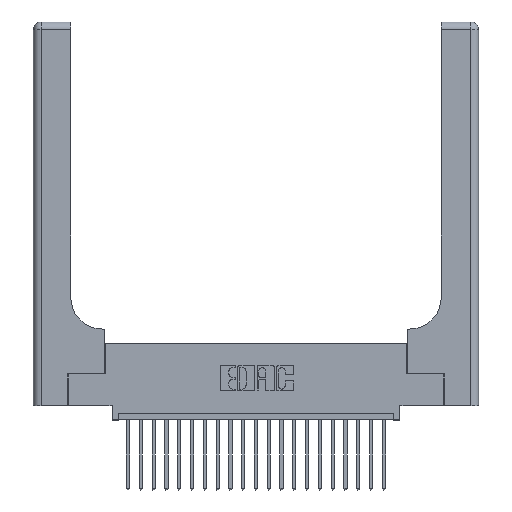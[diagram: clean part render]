
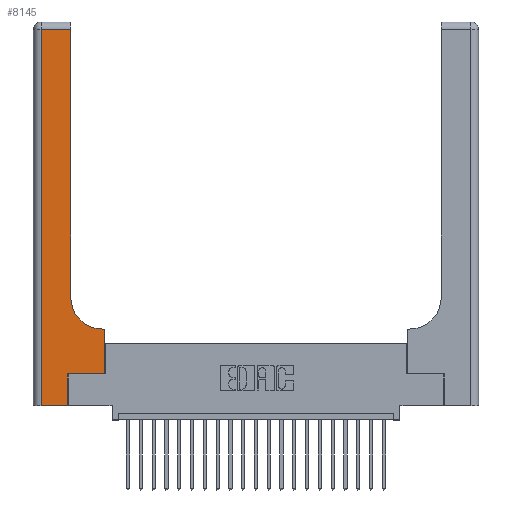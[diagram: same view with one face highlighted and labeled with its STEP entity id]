
A CAD part, top view. The second image highlights one B-rep face of the part: STEP entity #8145.
In plain terms, the highlighted planar face has unit normal (0, 0, 1).
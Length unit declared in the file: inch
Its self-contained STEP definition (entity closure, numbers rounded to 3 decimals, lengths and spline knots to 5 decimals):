
#532 = EDGE_CURVE ( 'NONE', #6200, #13840, #13976, .T. ) ;
#576 = VECTOR ( 'NONE', #5150, 39.37008 ) ;
#609 = CIRCLE ( 'NONE', #21544, 0.25 ) ;
#1213 = EDGE_CURVE ( 'NONE', #2058, #22626, #7510, .T. ) ;
#1431 = VECTOR ( 'NONE', #8332, 39.37008 ) ;
#1507 = DIRECTION ( 'NONE',  ( -1., 0., 0. ) ) ;
#1637 = CARTESIAN_POINT ( 'NONE',  ( 0.06, 0., 0.37 ) ) ;
#1995 = DIRECTION ( 'NONE',  ( 0., 1., 0. ) ) ;
#1996 = LINE ( 'NONE', #12170, #1431 ) ;
#2058 = VERTEX_POINT ( 'NONE', #10791 ) ;
#2705 = VECTOR ( 'NONE', #20865, 39.37008 ) ;
#3400 = DIRECTION ( 'NONE',  ( 0., -1., 0. ) ) ;
#3778 = EDGE_CURVE ( 'NONE', #13840, #16479, #17340, .T. ) ;
#4126 = FACE_OUTER_BOUND ( 'NONE', #4736, .T. ) ;
#4736 = EDGE_LOOP ( 'NONE', ( #5119, #21849, #23039, #14675, #19238, #20548, #11868, #14388, #14847 ) ) ;
#5119 = ORIENTED_EDGE ( 'NONE', *, *, #18127, .T. ) ;
#5150 = DIRECTION ( 'NONE',  ( 0., 1., 0. ) ) ;
#5796 = VECTOR ( 'NONE', #3400, 39.37008 ) ;
#5924 = CARTESIAN_POINT ( 'NONE',  ( 0.06, 2.94, 0.37 ) ) ;
#6200 = VERTEX_POINT ( 'NONE', #5924 ) ;
#6630 = DIRECTION ( 'NONE',  ( 1., 0., 0. ) ) ;
#7039 = CARTESIAN_POINT ( 'NONE',  ( 0.5585, 0.6, 0.37 ) ) ;
#7337 = VERTEX_POINT ( 'NONE', #23247 ) ;
#7508 = CARTESIAN_POINT ( 'NONE',  ( 0.06, 3., 0.37 ) ) ;
#7510 = LINE ( 'NONE', #7542, #11267 ) ;
#7542 = CARTESIAN_POINT ( 'NONE',  ( 0.5585, 0.25, 0.37 ) ) ;
#7878 = LINE ( 'NONE', #15792, #576 ) ;
#8145 = ADVANCED_FACE ( 'NONE', ( #4126 ), #12210, .F. ) ;
#8175 = VERTEX_POINT ( 'NONE', #12602 ) ;
#8332 = DIRECTION ( 'NONE',  ( -1., 0., 0. ) ) ;
#8670 = VECTOR ( 'NONE', #23509, 39.37008 ) ;
#9211 = VERTEX_POINT ( 'NONE', #11622 ) ;
#9389 = DIRECTION ( 'NONE',  ( 0., 1., 0. ) ) ;
#10196 = EDGE_CURVE ( 'NONE', #16479, #9211, #15954, .T. ) ;
#10234 = EDGE_CURVE ( 'NONE', #7337, #6200, #22549, .T. ) ;
#10723 = VECTOR ( 'NONE', #1507, 39.37008 ) ;
#10791 = CARTESIAN_POINT ( 'NONE',  ( 0.5585, 0.25, 0.37 ) ) ;
#10989 = VECTOR ( 'NONE', #1995, 39.37008 ) ;
#11267 = VECTOR ( 'NONE', #9389, 39.37008 ) ;
#11318 = CARTESIAN_POINT ( 'NONE',  ( 0.269, 0.25, 0.37 ) ) ;
#11323 = CARTESIAN_POINT ( 'NONE',  ( 0., 0., 0.37 ) ) ;
#11425 = CARTESIAN_POINT ( 'NONE',  ( 0.269, 0., 0.37 ) ) ;
#11622 = CARTESIAN_POINT ( 'NONE',  ( 0.269, 0.25, 0.37 ) ) ;
#11868 = ORIENTED_EDGE ( 'NONE', *, *, #1213, .T. ) ;
#11921 = AXIS2_PLACEMENT_3D ( 'NONE', #15779, #23682, #19747 ) ;
#12170 = CARTESIAN_POINT ( 'NONE',  ( 0.2915, 0.6, 0.37 ) ) ;
#12210 = PLANE ( 'NONE',  #11921 ) ;
#12602 = CARTESIAN_POINT ( 'NONE',  ( 0.2915, 0.85, 0.37 ) ) ;
#13005 = CARTESIAN_POINT ( 'NONE',  ( 0.269, 0., 0.37 ) ) ;
#13112 = EDGE_CURVE ( 'NONE', #9211, #2058, #22101, .T. ) ;
#13840 = VERTEX_POINT ( 'NONE', #1637 ) ;
#13976 = LINE ( 'NONE', #7508, #5796 ) ;
#14388 = ORIENTED_EDGE ( 'NONE', *, *, #19493, .T. ) ;
#14675 = ORIENTED_EDGE ( 'NONE', *, *, #3778, .T. ) ;
#14847 = ORIENTED_EDGE ( 'NONE', *, *, #23171, .T. ) ;
#15779 = CARTESIAN_POINT ( 'NONE',  ( 0., 3., 0.37 ) ) ;
#15792 = CARTESIAN_POINT ( 'NONE',  ( 0.2915, 3., 0.37 ) ) ;
#15954 = LINE ( 'NONE', #11425, #10989 ) ;
#16099 = CARTESIAN_POINT ( 'NONE',  ( 0.5415, 0.85, 0.37 ) ) ;
#16479 = VERTEX_POINT ( 'NONE', #13005 ) ;
#16600 = CARTESIAN_POINT ( 'NONE',  ( 0.5415, 0.6, 0.37 ) ) ;
#17340 = LINE ( 'NONE', #11323, #8670 ) ;
#18127 = EDGE_CURVE ( 'NONE', #8175, #7337, #7878, .T. ) ;
#19238 = ORIENTED_EDGE ( 'NONE', *, *, #10196, .T. ) ;
#19493 = EDGE_CURVE ( 'NONE', #22626, #21515, #1996, .T. ) ;
#19747 = DIRECTION ( 'NONE',  ( -1., 0., 0. ) ) ;
#20548 = ORIENTED_EDGE ( 'NONE', *, *, #13112, .T. ) ;
#20865 = DIRECTION ( 'NONE',  ( 1., 0., 0. ) ) ;
#21515 = VERTEX_POINT ( 'NONE', #16600 ) ;
#21544 = AXIS2_PLACEMENT_3D ( 'NONE', #16099, #23326, #6630 ) ;
#21672 = CARTESIAN_POINT ( 'NONE',  ( 0., 2.94, 0.37 ) ) ;
#21849 = ORIENTED_EDGE ( 'NONE', *, *, #10234, .T. ) ;
#22101 = LINE ( 'NONE', #11318, #2705 ) ;
#22549 = LINE ( 'NONE', #21672, #10723 ) ;
#22626 = VERTEX_POINT ( 'NONE', #7039 ) ;
#23039 = ORIENTED_EDGE ( 'NONE', *, *, #532, .T. ) ;
#23171 = EDGE_CURVE ( 'NONE', #21515, #8175, #609, .T. ) ;
#23247 = CARTESIAN_POINT ( 'NONE',  ( 0.2915, 2.94, 0.37 ) ) ;
#23326 = DIRECTION ( 'NONE',  ( 0., 0., -1. ) ) ;
#23509 = DIRECTION ( 'NONE',  ( 1., 0., 0. ) ) ;
#23682 = DIRECTION ( 'NONE',  ( 0., 0., -1. ) ) ;
